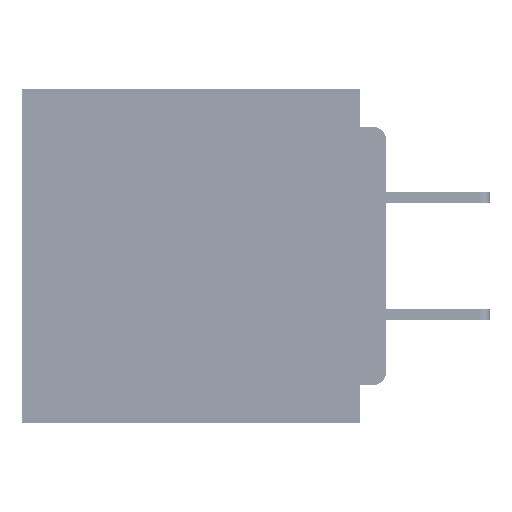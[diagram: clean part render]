
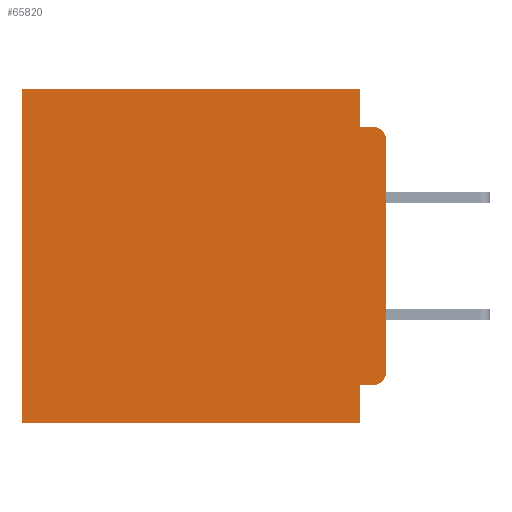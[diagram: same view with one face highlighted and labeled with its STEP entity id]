
A CAD part, left-side view. The second image highlights one B-rep face of the part: STEP entity #65820.
In plain terms, the highlighted planar face has unit normal (-1, 0, 0).
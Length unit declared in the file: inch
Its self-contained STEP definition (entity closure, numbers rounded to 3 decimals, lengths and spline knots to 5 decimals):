
#1014 = AXIS2_PLACEMENT_3D ( 'NONE', #58210, #26398, #63541 ) ;
#1679 = DIRECTION ( 'NONE',  ( -1., 0., 0. ) ) ;
#1926 = DIRECTION ( 'NONE',  ( 0., 0., -1. ) ) ;
#3157 = CARTESIAN_POINT ( 'NONE',  ( 0.3, 0.031, -0.355 ) ) ;
#4434 = VERTEX_POINT ( 'NONE', #3157 ) ;
#5345 = ORIENTED_EDGE ( 'NONE', *, *, #38045, .F. ) ;
#5779 = LINE ( 'NONE', #53578, #46560 ) ;
#6659 = VERTEX_POINT ( 'NONE', #11965 ) ;
#7106 = EDGE_CURVE ( 'NONE', #68073, #65282, #22620, .T. ) ;
#7206 = CARTESIAN_POINT ( 'NONE',  ( 0.3, 0., -0.4 ) ) ;
#7762 = ORIENTED_EDGE ( 'NONE', *, *, #39479, .T. ) ;
#9033 = EDGE_CURVE ( 'NONE', #65282, #12045, #5779, .T. ) ;
#9783 = CARTESIAN_POINT ( 'NONE',  ( 0.3, 0.015, -0.355 ) ) ;
#10523 = CARTESIAN_POINT ( 'NONE',  ( 0.3, 0., 0. ) ) ;
#11481 = FACE_OUTER_BOUND ( 'NONE', #42159, .T. ) ;
#11965 = CARTESIAN_POINT ( 'NONE',  ( 0.3, 0.015, -0.045 ) ) ;
#12045 = VERTEX_POINT ( 'NONE', #47081 ) ;
#12805 = CARTESIAN_POINT ( 'NONE',  ( 0.3, 0., -0.045 ) ) ;
#13800 = CARTESIAN_POINT ( 'NONE',  ( 0.3, 0.031, -0.4 ) ) ;
#15237 = ORIENTED_EDGE ( 'NONE', *, *, #7106, .T. ) ;
#15395 = CARTESIAN_POINT ( 'NONE',  ( 0.3, 0., -0.4 ) ) ;
#15416 = PLANE ( 'NONE',  #1014 ) ;
#15875 = CARTESIAN_POINT ( 'NONE',  ( 0.3, 0., -0.355 ) ) ;
#16029 = VERTEX_POINT ( 'NONE', #47016 ) ;
#16592 = AXIS2_PLACEMENT_3D ( 'NONE', #33497, #1679, #38856 ) ;
#19091 = DIRECTION ( 'NONE',  ( 0., -1., 0. ) ) ;
#19765 = VECTOR ( 'NONE', #41935, 39.37008 ) ;
#21419 = LINE ( 'NONE', #15875, #40564 ) ;
#21748 = DIRECTION ( 'NONE',  ( 0., 0., -1. ) ) ;
#22620 = LINE ( 'NONE', #10523, #49215 ) ;
#22649 = EDGE_CURVE ( 'NONE', #31947, #12045, #62198, .T. ) ;
#23476 = VECTOR ( 'NONE', #51025, 39.37008 ) ;
#24244 = VERTEX_POINT ( 'NONE', #32754 ) ;
#26398 = DIRECTION ( 'NONE',  ( 1., 0., 0. ) ) ;
#27944 = EDGE_CURVE ( 'NONE', #24244, #6659, #54911, .T. ) ;
#29364 = LINE ( 'NONE', #59477, #55964 ) ;
#30057 = VERTEX_POINT ( 'NONE', #34564 ) ;
#30722 = ORIENTED_EDGE ( 'NONE', *, *, #55143, .F. ) ;
#31938 = DIRECTION ( 'NONE',  ( 0., 1., 0. ) ) ;
#31947 = VERTEX_POINT ( 'NONE', #35740 ) ;
#32754 = CARTESIAN_POINT ( 'NONE',  ( 0.3, 0.031, -0.045 ) ) ;
#33497 = CARTESIAN_POINT ( 'NONE',  ( 0.3, 0.015, -0.06 ) ) ;
#33763 = DIRECTION ( 'NONE',  ( -1., 0., 0. ) ) ;
#34564 = CARTESIAN_POINT ( 'NONE',  ( 0.3, 0., -0.06 ) ) ;
#34946 = CIRCLE ( 'NONE', #16592, 0.015 ) ;
#35041 = EDGE_CURVE ( 'NONE', #59971, #16029, #54493, .T. ) ;
#35740 = CARTESIAN_POINT ( 'NONE',  ( 0.3, 0.031, -0.4 ) ) ;
#35880 = ORIENTED_EDGE ( 'NONE', *, *, #9033, .T. ) ;
#37611 = EDGE_CURVE ( 'NONE', #30057, #16029, #61032, .T. ) ;
#38045 = EDGE_CURVE ( 'NONE', #68073, #24244, #29364, .T. ) ;
#38856 = DIRECTION ( 'NONE',  ( 0., 0., -1. ) ) ;
#39479 = EDGE_CURVE ( 'NONE', #30057, #6659, #34946, .T. ) ;
#40564 = VECTOR ( 'NONE', #31938, 39.37008 ) ;
#41935 = DIRECTION ( 'NONE',  ( 0., 1., 0. ) ) ;
#42159 = EDGE_LOOP ( 'NONE', ( #47885, #7762, #45078, #5345, #15237, #35880, #48185, #43099, #30722, #62937 ) ) ;
#42398 = DIRECTION ( 'NONE',  ( 0., 1., 0. ) ) ;
#43099 = ORIENTED_EDGE ( 'NONE', *, *, #59153, .F. ) ;
#45078 = ORIENTED_EDGE ( 'NONE', *, *, #27944, .F. ) ;
#45208 = VECTOR ( 'NONE', #65554, 39.37008 ) ;
#46560 = VECTOR ( 'NONE', #21748, 39.37008 ) ;
#47016 = CARTESIAN_POINT ( 'NONE',  ( 0.3, 0., -0.34 ) ) ;
#47081 = CARTESIAN_POINT ( 'NONE',  ( 0.3, 0.437, -0.4 ) ) ;
#47885 = ORIENTED_EDGE ( 'NONE', *, *, #37611, .F. ) ;
#48185 = ORIENTED_EDGE ( 'NONE', *, *, #22649, .F. ) ;
#49215 = VECTOR ( 'NONE', #42398, 39.37008 ) ;
#51025 = DIRECTION ( 'NONE',  ( 0., 0., -1. ) ) ;
#53232 = VECTOR ( 'NONE', #19091, 39.37008 ) ;
#53578 = CARTESIAN_POINT ( 'NONE',  ( 0.3, 0.437, -0.4 ) ) ;
#54493 = CIRCLE ( 'NONE', #66306, 0.015 ) ;
#54911 = LINE ( 'NONE', #12805, #53232 ) ;
#55143 = EDGE_CURVE ( 'NONE', #59971, #4434, #21419, .T. ) ;
#55964 = VECTOR ( 'NONE', #64829, 39.37008 ) ;
#58210 = CARTESIAN_POINT ( 'NONE',  ( 0.3, 0., -0.4 ) ) ;
#58295 = CARTESIAN_POINT ( 'NONE',  ( 0.3, 0.437, 0. ) ) ;
#59153 = EDGE_CURVE ( 'NONE', #4434, #31947, #65846, .T. ) ;
#59477 = CARTESIAN_POINT ( 'NONE',  ( 0.3, 0.031, 0. ) ) ;
#59971 = VERTEX_POINT ( 'NONE', #9783 ) ;
#61032 = LINE ( 'NONE', #7206, #45208 ) ;
#61945 = CARTESIAN_POINT ( 'NONE',  ( 0.3, 0.031, 0. ) ) ;
#62198 = LINE ( 'NONE', #15395, #19765 ) ;
#62937 = ORIENTED_EDGE ( 'NONE', *, *, #35041, .T. ) ;
#63541 = DIRECTION ( 'NONE',  ( 0., 0., -1. ) ) ;
#64829 = DIRECTION ( 'NONE',  ( 0., 0., -1. ) ) ;
#65282 = VERTEX_POINT ( 'NONE', #58295 ) ;
#65554 = DIRECTION ( 'NONE',  ( 0., 0., -1. ) ) ;
#65594 = CARTESIAN_POINT ( 'NONE',  ( 0.3, 0.015, -0.34 ) ) ;
#65820 = ADVANCED_FACE ( 'NONE', ( #11481 ), #15416, .F. ) ;
#65846 = LINE ( 'NONE', #13800, #23476 ) ;
#66306 = AXIS2_PLACEMENT_3D ( 'NONE', #65594, #33763, #1926 ) ;
#68073 = VERTEX_POINT ( 'NONE', #61945 ) ;
